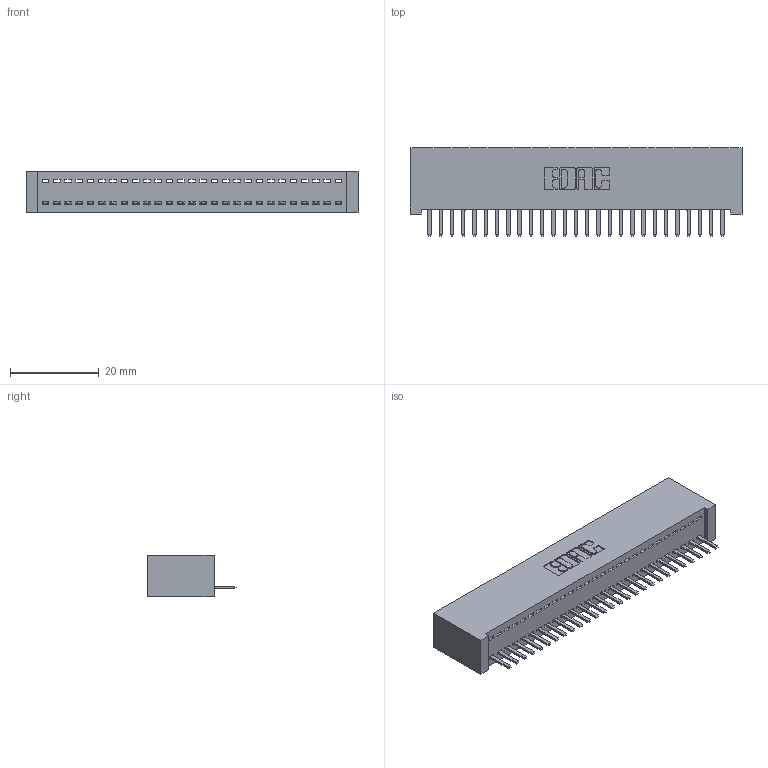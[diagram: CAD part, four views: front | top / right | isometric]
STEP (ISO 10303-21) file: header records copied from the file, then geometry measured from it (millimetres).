
FILE_DESCRIPTION (( 'STEP AP203' ), '1' );
FILE_NAME ('392-027-520-101.STEP', '2018-08-15T20:17:58', ( '' ), ( '' ), 'SwSTEP 2.0', 'SolidWorks 2016', '' );
FILE_SCHEMA (( 'CONFIG_CONTROL_DESIGN' ));
Length unit declared in the file: inch
Products named in the file (3): 342 Part_Lugless; 345-292-001_345-293-120; 392-027-520-101
Assembly tree (28 placements, depth 2):
  392-027-520-101
    342 Part_Lugless
    345-292-001_345-293-120  x27
Bounding box: 74.83 x 20.02 x 9.4 mm (x, y, z)
Volume: 6837 mm3; surface area: 9834.7 mm2
Topology: 28 solids, 28 shells, 1776 faces, 5243 edges, 3422 vertices
Faces by surface type: plane 1250, cylinder 526
Entity records: 18151 total; most frequent: CARTESIAN_POINT 3151, ORIENTED_EDGE 3102, DIRECTION 2669, EDGE_CURVE 1551, LINE 1427, VECTOR 1427, VERTEX_POINT 1030, AXIS2_PLACEMENT_3D 621
